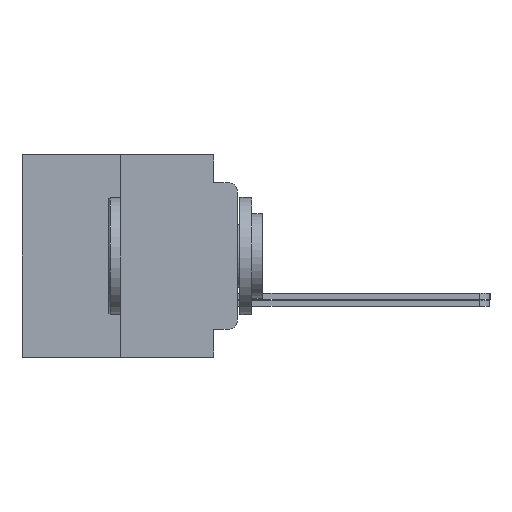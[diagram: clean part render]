
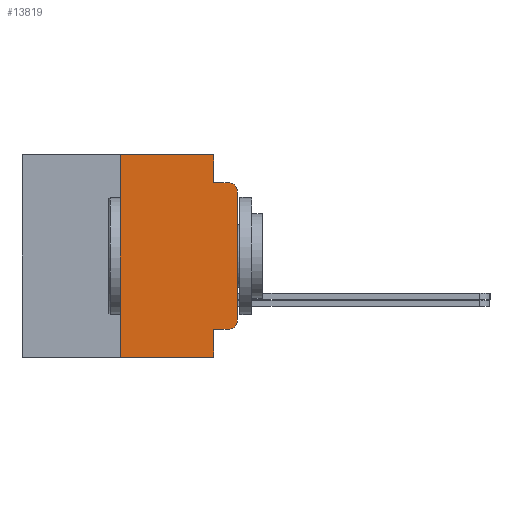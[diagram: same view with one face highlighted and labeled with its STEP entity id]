
A CAD part, left-side view. The second image highlights one B-rep face of the part: STEP entity #13819.
In plain terms, the highlighted planar face has unit normal (-1, 0, 0).
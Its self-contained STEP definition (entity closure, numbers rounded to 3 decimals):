
#68 = AXIS2_PLACEMENT_3D ( 'NONE', #27750, #9900, #1252 ) ;
#232 = CARTESIAN_POINT ( 'NONE',  ( -75.603, 11.684, 5.486 ) ) ;
#454 = LINE ( 'NONE', #232, #17311 ) ;
#697 = VERTEX_POINT ( 'NONE', #15372 ) ;
#881 = EDGE_CURVE ( 'NONE', #27331, #19937, #13708, .T. ) ;
#920 = DIRECTION ( 'NONE',  ( 0., 0., -1. ) ) ;
#1110 = EDGE_CURVE ( 'NONE', #7643, #9331, #1623, .T. ) ;
#1252 = DIRECTION ( 'NONE',  ( 0., 0., -1. ) ) ;
#1623 = LINE ( 'NONE', #3580, #14703 ) ;
#1683 = CARTESIAN_POINT ( 'NONE',  ( -75.603, 1.295, -3.975 ) ) ;
#1738 = VERTEX_POINT ( 'NONE', #13766 ) ;
#1776 = EDGE_CURVE ( 'NONE', #1738, #697, #13283, .T. ) ;
#2375 = CARTESIAN_POINT ( 'NONE',  ( -75.603, 0.508, -3.975 ) ) ;
#2544 = DIRECTION ( 'NONE',  ( 0., -1., 0. ) ) ;
#2674 = CARTESIAN_POINT ( 'NONE',  ( -75.603, 1.295, 5.486 ) ) ;
#2836 = AXIS2_PLACEMENT_3D ( 'NONE', #7732, #10028, #25531 ) ;
#3400 = PLANE ( 'NONE',  #2836 ) ;
#3580 = CARTESIAN_POINT ( 'NONE',  ( -75.603, 1.295, 0. ) ) ;
#3617 = CARTESIAN_POINT ( 'NONE',  ( -75.603, 0., 5.486 ) ) ;
#4244 = CARTESIAN_POINT ( 'NONE',  ( -75.603, 0., 3.467 ) ) ;
#4818 = ORIENTED_EDGE ( 'NONE', *, *, #881, .F. ) ;
#4925 = EDGE_CURVE ( 'NONE', #7643, #28515, #17920, .T. ) ;
#4941 = VERTEX_POINT ( 'NONE', #28156 ) ;
#5258 = DIRECTION ( 'NONE',  ( -1., 0., 0. ) ) ;
#6485 = CARTESIAN_POINT ( 'NONE',  ( -75.603, 1.295, 0. ) ) ;
#6693 = ORIENTED_EDGE ( 'NONE', *, *, #25603, .F. ) ;
#7643 = VERTEX_POINT ( 'NONE', #17384 ) ;
#7732 = CARTESIAN_POINT ( 'NONE',  ( -75.603, 11.684, 5.486 ) ) ;
#8017 = EDGE_CURVE ( 'NONE', #19578, #697, #10971, .T. ) ;
#8134 = DIRECTION ( 'NONE',  ( 0., 0., 1. ) ) ;
#8239 = LINE ( 'NONE', #6485, #13059 ) ;
#8263 = LINE ( 'NONE', #3617, #19290 ) ;
#8429 = ORIENTED_EDGE ( 'NONE', *, *, #16151, .F. ) ;
#9098 = FACE_OUTER_BOUND ( 'NONE', #24935, .T. ) ;
#9331 = VERTEX_POINT ( 'NONE', #12792 ) ;
#9900 = DIRECTION ( 'NONE',  ( -1., 0., 0. ) ) ;
#10028 = DIRECTION ( 'NONE',  ( 1., 0., 0. ) ) ;
#10971 = CIRCLE ( 'NONE', #12988, 0.508 ) ;
#11434 = CARTESIAN_POINT ( 'NONE',  ( -75.603, 1.295, 3.975 ) ) ;
#11692 = ORIENTED_EDGE ( 'NONE', *, *, #22982, .T. ) ;
#12317 = CARTESIAN_POINT ( 'NONE',  ( -75.603, 6.35, -5.486 ) ) ;
#12657 = CARTESIAN_POINT ( 'NONE',  ( -75.603, 6.35, -5.486 ) ) ;
#12792 = CARTESIAN_POINT ( 'NONE',  ( -75.603, 1.295, -5.486 ) ) ;
#12943 = VECTOR ( 'NONE', #24683, 1000. ) ;
#12988 = AXIS2_PLACEMENT_3D ( 'NONE', #27304, #5258, #920 ) ;
#13019 = VERTEX_POINT ( 'NONE', #2674 ) ;
#13059 = VECTOR ( 'NONE', #21911, 1000. ) ;
#13283 = LINE ( 'NONE', #11434, #12943 ) ;
#13708 = LINE ( 'NONE', #12317, #23744 ) ;
#13766 = CARTESIAN_POINT ( 'NONE',  ( -75.603, 1.295, 3.975 ) ) ;
#13819 = ADVANCED_FACE ( 'NONE', ( #9098 ), #3400, .F. ) ;
#14553 = DIRECTION ( 'NONE',  ( 0., -1., 0. ) ) ;
#14703 = VECTOR ( 'NONE', #23179, 1000. ) ;
#15372 = CARTESIAN_POINT ( 'NONE',  ( -75.603, 0.508, 3.975 ) ) ;
#16151 = EDGE_CURVE ( 'NONE', #19937, #13019, #454, .T. ) ;
#16629 = ORIENTED_EDGE ( 'NONE', *, *, #1776, .F. ) ;
#17311 = VECTOR ( 'NONE', #2544, 1000. ) ;
#17384 = CARTESIAN_POINT ( 'NONE',  ( -75.603, 1.295, -3.975 ) ) ;
#17920 = LINE ( 'NONE', #1683, #27297 ) ;
#18209 = ORIENTED_EDGE ( 'NONE', *, *, #8017, .T. ) ;
#19290 = VECTOR ( 'NONE', #8134, 1000. ) ;
#19578 = VERTEX_POINT ( 'NONE', #4244 ) ;
#19937 = VERTEX_POINT ( 'NONE', #25108 ) ;
#21911 = DIRECTION ( 'NONE',  ( 0., 0., -1. ) ) ;
#22249 = ORIENTED_EDGE ( 'NONE', *, *, #4925, .T. ) ;
#22589 = ORIENTED_EDGE ( 'NONE', *, *, #26079, .T. ) ;
#22982 = EDGE_CURVE ( 'NONE', #28515, #4941, #26681, .T. ) ;
#23179 = DIRECTION ( 'NONE',  ( 0., 0., -1. ) ) ;
#23744 = VECTOR ( 'NONE', #25401, 1000. ) ;
#24683 = DIRECTION ( 'NONE',  ( 0., -1., 0. ) ) ;
#24935 = EDGE_LOOP ( 'NONE', ( #22249, #11692, #26792, #18209, #16629, #6693, #8429, #4818, #22589, #26261 ) ) ;
#25108 = CARTESIAN_POINT ( 'NONE',  ( -75.603, 6.35, 5.486 ) ) ;
#25401 = DIRECTION ( 'NONE',  ( 0., 0., 1. ) ) ;
#25445 = EDGE_CURVE ( 'NONE', #4941, #19578, #8263, .T. ) ;
#25531 = DIRECTION ( 'NONE',  ( 0., 0., -1. ) ) ;
#25603 = EDGE_CURVE ( 'NONE', #13019, #1738, #8239, .T. ) ;
#26049 = DIRECTION ( 'NONE',  ( 0., -1., 0. ) ) ;
#26079 = EDGE_CURVE ( 'NONE', #27331, #9331, #27625, .T. ) ;
#26261 = ORIENTED_EDGE ( 'NONE', *, *, #1110, .F. ) ;
#26681 = CIRCLE ( 'NONE', #68, 0.508 ) ;
#26792 = ORIENTED_EDGE ( 'NONE', *, *, #25445, .T. ) ;
#27297 = VECTOR ( 'NONE', #26049, 1000. ) ;
#27304 = CARTESIAN_POINT ( 'NONE',  ( -75.603, 0.508, 3.467 ) ) ;
#27331 = VERTEX_POINT ( 'NONE', #12657 ) ;
#27625 = LINE ( 'NONE', #27940, #28301 ) ;
#27750 = CARTESIAN_POINT ( 'NONE',  ( -75.603, 0.508, -3.467 ) ) ;
#27940 = CARTESIAN_POINT ( 'NONE',  ( -75.603, 11.684, -5.486 ) ) ;
#28156 = CARTESIAN_POINT ( 'NONE',  ( -75.603, 0., -3.467 ) ) ;
#28301 = VECTOR ( 'NONE', #14553, 1000. ) ;
#28515 = VERTEX_POINT ( 'NONE', #2375 ) ;
